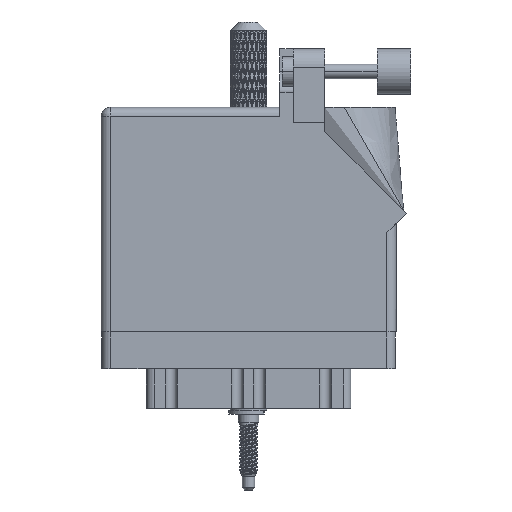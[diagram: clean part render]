
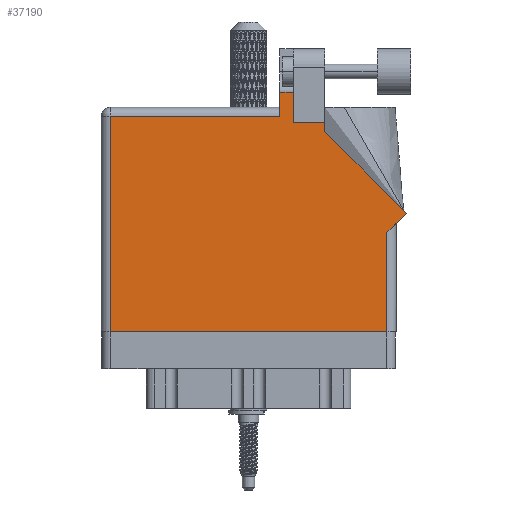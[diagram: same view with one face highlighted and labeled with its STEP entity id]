
A CAD part, front view. The second image highlights one B-rep face of the part: STEP entity #37190.
In plain terms, the highlighted face is planar.
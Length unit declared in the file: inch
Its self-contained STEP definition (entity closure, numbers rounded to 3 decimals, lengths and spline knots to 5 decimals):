
#1737 = VERTEX_POINT ( 'NONE', #99269 ) ;
#1810 = CARTESIAN_POINT ( 'NONE',  ( 1.64177, 1.6315, 0. ) ) ;
#2926 = EDGE_CURVE ( 'NONE', #104514, #71207, #17229, .T. ) ;
#3032 = ORIENTED_EDGE ( 'NONE', *, *, #79450, .T. ) ;
#3414 = EDGE_CURVE ( 'NONE', #1737, #46832, #87871, .T. ) ;
#3516 = CARTESIAN_POINT ( 'NONE',  ( 2.08071, 0.80771, 0. ) ) ;
#8266 = VERTEX_POINT ( 'NONE', #87705 ) ;
#8441 = DIRECTION ( 'NONE',  ( -1., 0., 0. ) ) ;
#10769 = EDGE_CURVE ( 'NONE', #50083, #62614, #28977, .T. ) ;
#11314 = VECTOR ( 'NONE', #50574, 39.37008 ) ;
#14342 = CARTESIAN_POINT ( 'NONE',  ( 1.524, 1.43, 0. ) ) ;
#14606 = VECTOR ( 'NONE', #18082, 39.37008 ) ;
#15140 = CARTESIAN_POINT ( 'NONE',  ( 0., 0., 0. ) ) ;
#17229 = LINE ( 'NONE', #1810, #23404 ) ;
#17749 = DIRECTION ( 'NONE',  ( -1., 0., 0. ) ) ;
#18082 = DIRECTION ( 'NONE',  ( 0., -1., 0. ) ) ;
#19517 = ORIENTED_EDGE ( 'NONE', *, *, #10769, .T. ) ;
#23404 = VECTOR ( 'NONE', #17749, 39.37008 ) ;
#23594 = ORIENTED_EDGE ( 'NONE', *, *, #52870, .T. ) ;
#24617 = ORIENTED_EDGE ( 'NONE', *, *, #96082, .T. ) ;
#25361 = ORIENTED_EDGE ( 'NONE', *, *, #3414, .T. ) ;
#26089 = EDGE_CURVE ( 'NONE', #40266, #100058, #88381, .T. ) ;
#28482 = VECTOR ( 'NONE', #47523, 39.37008 ) ;
#28977 = LINE ( 'NONE', #36385, #29772 ) ;
#29772 = VECTOR ( 'NONE', #85240, 39.37008 ) ;
#30330 = CARTESIAN_POINT ( 'NONE',  ( 0.062, 1.468, 0. ) ) ;
#32562 = LINE ( 'NONE', #64432, #45939 ) ;
#36352 = EDGE_LOOP ( 'NONE', ( #97293, #76550, #23594, #19517, #50608, #25361, #3032, #47866, #76600, #95364, #24617 ) ) ;
#36372 = PLANE ( 'NONE',  #104439 ) ;
#36385 = CARTESIAN_POINT ( 'NONE',  ( 0., 1.468, 0. ) ) ;
#37190 = ADVANCED_FACE ( 'NONE', ( #84702 ), #36372, .F. ) ;
#39018 = CARTESIAN_POINT ( 'NONE',  ( 2.01, 0.737, 0. ) ) ;
#40266 = VERTEX_POINT ( 'NONE', #76484 ) ;
#44352 = DIRECTION ( 'NONE',  ( -1., 0., 0. ) ) ;
#44867 = CARTESIAN_POINT ( 'NONE',  ( 0., 1.53, 0. ) ) ;
#45939 = VECTOR ( 'NONE', #90383, 39.37008 ) ;
#46832 = VERTEX_POINT ( 'NONE', #84682 ) ;
#47523 = DIRECTION ( 'NONE',  ( 1., 0., 0. ) ) ;
#47554 = CARTESIAN_POINT ( 'NONE',  ( 1.311, 1.43, 0. ) ) ;
#47866 = ORIENTED_EDGE ( 'NONE', *, *, #26089, .T. ) ;
#49629 = VERTEX_POINT ( 'NONE', #81196 ) ;
#49949 = LINE ( 'NONE', #65360, #14606 ) ;
#50083 = VERTEX_POINT ( 'NONE', #76218 ) ;
#50574 = DIRECTION ( 'NONE',  ( 0., 1., 0. ) ) ;
#50608 = ORIENTED_EDGE ( 'NONE', *, *, #92107, .T. ) ;
#52104 = VECTOR ( 'NONE', #78043, 39.37008 ) ;
#52870 = EDGE_CURVE ( 'NONE', #71207, #50083, #99225, .T. ) ;
#53045 = CARTESIAN_POINT ( 'NONE',  ( 1.524, 1.43, 0. ) ) ;
#55732 = CARTESIAN_POINT ( 'NONE',  ( 2.08071, 0.80771, 0. ) ) ;
#57497 = CARTESIAN_POINT ( 'NONE',  ( 1.524, 1.36442, 0. ) ) ;
#58523 = LINE ( 'NONE', #57497, #11314 ) ;
#62614 = VERTEX_POINT ( 'NONE', #30330 ) ;
#64432 = CARTESIAN_POINT ( 'NONE',  ( 1.948, 0.737, 0. ) ) ;
#64500 = DIRECTION ( 'NONE',  ( 0.707, 0.707, 0. ) ) ;
#65360 = CARTESIAN_POINT ( 'NONE',  ( 0.062, 0., 0. ) ) ;
#66355 = EDGE_CURVE ( 'NONE', #49629, #88563, #58523, .T. ) ;
#71207 = VERTEX_POINT ( 'NONE', #75152 ) ;
#73012 = VECTOR ( 'NONE', #94784, 39.37008 ) ;
#75152 = CARTESIAN_POINT ( 'NONE',  ( 1.217, 1.6315, 0. ) ) ;
#76218 = CARTESIAN_POINT ( 'NONE',  ( 1.217, 1.468, 0. ) ) ;
#76484 = CARTESIAN_POINT ( 'NONE',  ( 1.948, 0.675, 0. ) ) ;
#76550 = ORIENTED_EDGE ( 'NONE', *, *, #2926, .T. ) ;
#76600 = ORIENTED_EDGE ( 'NONE', *, *, #98564, .T. ) ;
#78043 = DIRECTION ( 'NONE',  ( -0.707, 0.707, 0. ) ) ;
#79450 = EDGE_CURVE ( 'NONE', #46832, #40266, #32562, .T. ) ;
#81196 = CARTESIAN_POINT ( 'NONE',  ( 1.524, 1.36442, 0. ) ) ;
#84682 = CARTESIAN_POINT ( 'NONE',  ( 1.948, 0., 0. ) ) ;
#84702 = FACE_OUTER_BOUND ( 'NONE', #36352, .T. ) ;
#85240 = DIRECTION ( 'NONE',  ( -1., 0., 0. ) ) ;
#86019 = VECTOR ( 'NONE', #64500, 39.37008 ) ;
#87705 = CARTESIAN_POINT ( 'NONE',  ( 1.311, 1.43, 0. ) ) ;
#87871 = LINE ( 'NONE', #15140, #28482 ) ;
#87896 = LINE ( 'NONE', #47554, #97356 ) ;
#88184 = EDGE_CURVE ( 'NONE', #8266, #104514, #87896, .T. ) ;
#88381 = LINE ( 'NONE', #39018, #86019 ) ;
#88563 = VERTEX_POINT ( 'NONE', #53045 ) ;
#88601 = CARTESIAN_POINT ( 'NONE',  ( 1.311, 1.6315, 0. ) ) ;
#90383 = DIRECTION ( 'NONE',  ( 0., 1., 0. ) ) ;
#91245 = CARTESIAN_POINT ( 'NONE',  ( 1.217, 1.53, 0. ) ) ;
#92107 = EDGE_CURVE ( 'NONE', #62614, #1737, #49949, .T. ) ;
#93709 = DIRECTION ( 'NONE',  ( 0., 0., -1. ) ) ;
#94784 = DIRECTION ( 'NONE',  ( 0., -1., 0. ) ) ;
#95364 = ORIENTED_EDGE ( 'NONE', *, *, #66355, .T. ) ;
#96082 = EDGE_CURVE ( 'NONE', #88563, #8266, #97120, .T. ) ;
#96371 = DIRECTION ( 'NONE',  ( 0., 1., 0. ) ) ;
#97120 = LINE ( 'NONE', #14342, #101297 ) ;
#97293 = ORIENTED_EDGE ( 'NONE', *, *, #88184, .T. ) ;
#97356 = VECTOR ( 'NONE', #96371, 39.37008 ) ;
#98564 = EDGE_CURVE ( 'NONE', #100058, #49629, #103001, .T. ) ;
#99225 = LINE ( 'NONE', #91245, #73012 ) ;
#99269 = CARTESIAN_POINT ( 'NONE',  ( 0.062, 0., 0. ) ) ;
#100058 = VERTEX_POINT ( 'NONE', #3516 ) ;
#101297 = VECTOR ( 'NONE', #8441, 39.37008 ) ;
#103001 = LINE ( 'NONE', #55732, #52104 ) ;
#104439 = AXIS2_PLACEMENT_3D ( 'NONE', #44867, #93709, #44352 ) ;
#104514 = VERTEX_POINT ( 'NONE', #88601 ) ;
